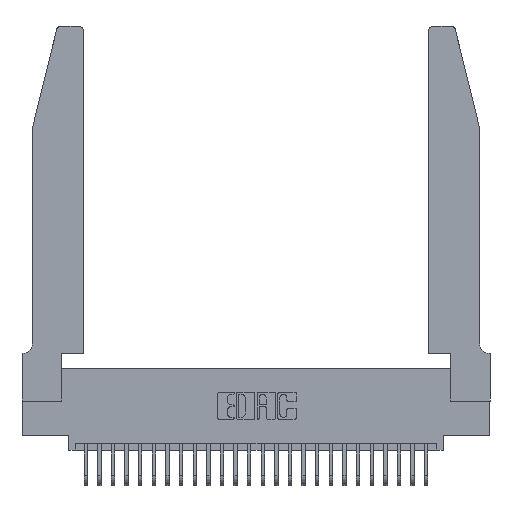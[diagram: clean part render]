
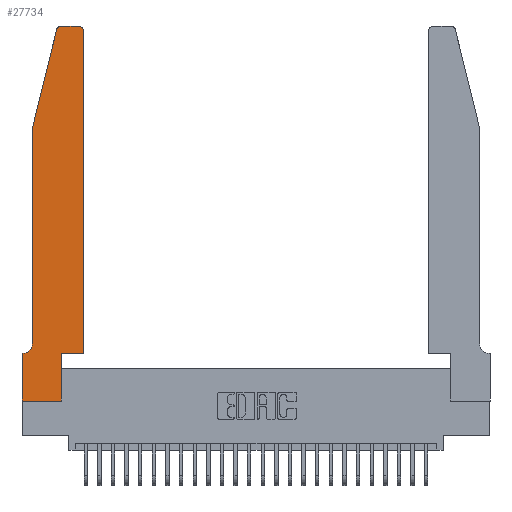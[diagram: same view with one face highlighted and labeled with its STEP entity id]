
A CAD part, top view. The second image highlights one B-rep face of the part: STEP entity #27734.
In plain terms, the highlighted planar face has unit normal (0, 0, 1).
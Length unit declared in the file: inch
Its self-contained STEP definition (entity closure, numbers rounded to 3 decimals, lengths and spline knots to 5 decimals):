
#188 = EDGE_CURVE ( 'NONE', #1949, #13038, #5815, .T. ) ;
#368 = LINE ( 'NONE', #1535, #14777 ) ;
#402 = CARTESIAN_POINT ( 'NONE',  ( 0.284, 2.75, 0.37 ) ) ;
#468 = AXIS2_PLACEMENT_3D ( 'NONE', #26087, #23922, #5599 ) ;
#580 = VERTEX_POINT ( 'NONE', #15066 ) ;
#971 = EDGE_LOOP ( 'NONE', ( #29012, #3470, #9494, #10318, #1989, #13173, #22170, #10500, #11775, #2356, #22865, #12247 ) ) ;
#1535 = CARTESIAN_POINT ( 'NONE',  ( 0., 0., 0.37 ) ) ;
#1949 = VERTEX_POINT ( 'NONE', #21469 ) ;
#1989 = ORIENTED_EDGE ( 'NONE', *, *, #4309, .T. ) ;
#2356 = ORIENTED_EDGE ( 'NONE', *, *, #188, .T. ) ;
#2629 = VERTEX_POINT ( 'NONE', #17180 ) ;
#3470 = ORIENTED_EDGE ( 'NONE', *, *, #5181, .T. ) ;
#3685 = LINE ( 'NONE', #28762, #26917 ) ;
#4158 = CARTESIAN_POINT ( 'NONE',  ( 0.0755, 2., 0.37 ) ) ;
#4309 = EDGE_CURVE ( 'NONE', #28322, #2629, #20389, .T. ) ;
#4954 = LINE ( 'NONE', #6471, #23658 ) ;
#5181 = EDGE_CURVE ( 'NONE', #15229, #28663, #14714, .T. ) ;
#5599 = DIRECTION ( 'NONE',  ( 1., 0., 0. ) ) ;
#5815 = LINE ( 'NONE', #12163, #25222 ) ;
#5998 = LINE ( 'NONE', #17079, #19383 ) ;
#6321 = DIRECTION ( 'NONE',  ( 0., 1., 0. ) ) ;
#6471 = CARTESIAN_POINT ( 'NONE',  ( 0.2605, 2.75, 0.37 ) ) ;
#6510 = CARTESIAN_POINT ( 'NONE',  ( 0.4205, 2.75, 0.37 ) ) ;
#6625 = EDGE_CURVE ( 'NONE', #580, #1949, #25628, .T. ) ;
#6723 = VECTOR ( 'NONE', #28165, 39.37008 ) ;
#7209 = CARTESIAN_POINT ( 'NONE',  ( 0.4205, 2.72, 0.37 ) ) ;
#8402 = EDGE_CURVE ( 'NONE', #13038, #26579, #3685, .T. ) ;
#8493 = FACE_OUTER_BOUND ( 'NONE', #971, .T. ) ;
#9494 = ORIENTED_EDGE ( 'NONE', *, *, #10702, .T. ) ;
#9653 = LINE ( 'NONE', #10586, #14929 ) ;
#10318 = ORIENTED_EDGE ( 'NONE', *, *, #11424, .T. ) ;
#10500 = ORIENTED_EDGE ( 'NONE', *, *, #14717, .T. ) ;
#10586 = CARTESIAN_POINT ( 'NONE',  ( 0., 0., 0.37 ) ) ;
#10702 = EDGE_CURVE ( 'NONE', #28663, #10866, #26811, .T. ) ;
#10866 = VERTEX_POINT ( 'NONE', #4158 ) ;
#11424 = EDGE_CURVE ( 'NONE', #10866, #28322, #5998, .T. ) ;
#11775 = ORIENTED_EDGE ( 'NONE', *, *, #6625, .T. ) ;
#11971 = DIRECTION ( 'NONE',  ( 0., 1., 0. ) ) ;
#12163 = CARTESIAN_POINT ( 'NONE',  ( 0.4505, 0.35, 0.37 ) ) ;
#12247 = ORIENTED_EDGE ( 'NONE', *, *, #17225, .T. ) ;
#12676 = CARTESIAN_POINT ( 'NONE',  ( 0.0755, 0.42, 0.37 ) ) ;
#13038 = VERTEX_POINT ( 'NONE', #16022 ) ;
#13173 = ORIENTED_EDGE ( 'NONE', *, *, #20077, .T. ) ;
#13421 = AXIS2_PLACEMENT_3D ( 'NONE', #7209, #18740, #27597 ) ;
#14231 = VERTEX_POINT ( 'NONE', #6510 ) ;
#14714 = CIRCLE ( 'NONE', #24878, 0.03 ) ;
#14717 = EDGE_CURVE ( 'NONE', #21330, #580, #368, .T. ) ;
#14777 = VECTOR ( 'NONE', #17518, 39.37008 ) ;
#14929 = VECTOR ( 'NONE', #19219, 39.37008 ) ;
#15066 = CARTESIAN_POINT ( 'NONE',  ( 0.2865, 0., 0.37 ) ) ;
#15229 = VERTEX_POINT ( 'NONE', #402 ) ;
#15526 = DIRECTION ( 'NONE',  ( -1., 0., 0. ) ) ;
#15791 = DIRECTION ( 'NONE',  ( 0., 0., 1. ) ) ;
#16022 = CARTESIAN_POINT ( 'NONE',  ( 0.4505, 0.35, 0.37 ) ) ;
#16034 = VERTEX_POINT ( 'NONE', #25802 ) ;
#16269 = DIRECTION ( 'NONE',  ( 1., 0., 0. ) ) ;
#17079 = CARTESIAN_POINT ( 'NONE',  ( 0.0755, 2., 0.37 ) ) ;
#17180 = CARTESIAN_POINT ( 'NONE',  ( 0.0055, 0.35, 0.37 ) ) ;
#17225 = EDGE_CURVE ( 'NONE', #26579, #14231, #18192, .T. ) ;
#17518 = DIRECTION ( 'NONE',  ( 1., 0., 0. ) ) ;
#18192 = CIRCLE ( 'NONE', #13421, 0.03 ) ;
#18740 = DIRECTION ( 'NONE',  ( 0., 0., 1. ) ) ;
#19219 = DIRECTION ( 'NONE',  ( 0., -1., 0. ) ) ;
#19383 = VECTOR ( 'NONE', #21771, 39.37008 ) ;
#19688 = LINE ( 'NONE', #27472, #22152 ) ;
#20077 = EDGE_CURVE ( 'NONE', #2629, #16034, #19688, .T. ) ;
#20389 = CIRCLE ( 'NONE', #21838, 0.07 ) ;
#20539 = CARTESIAN_POINT ( 'NONE',  ( 0.0755, 2., 0.37 ) ) ;
#20671 = VECTOR ( 'NONE', #11971, 39.37008 ) ;
#21330 = VERTEX_POINT ( 'NONE', #27000 ) ;
#21469 = CARTESIAN_POINT ( 'NONE',  ( 0.2865, 0.35, 0.37 ) ) ;
#21521 = DIRECTION ( 'NONE',  ( -1., 0., 0. ) ) ;
#21628 = CARTESIAN_POINT ( 'NONE',  ( 0.0055, 0.42, 0.37 ) ) ;
#21771 = DIRECTION ( 'NONE',  ( 0., -1., 0. ) ) ;
#21838 = AXIS2_PLACEMENT_3D ( 'NONE', #21628, #24008, #21521 ) ;
#22152 = VECTOR ( 'NONE', #25044, 39.37008 ) ;
#22170 = ORIENTED_EDGE ( 'NONE', *, *, #26011, .T. ) ;
#22609 = DIRECTION ( 'NONE',  ( 1., 0., 0. ) ) ;
#22865 = ORIENTED_EDGE ( 'NONE', *, *, #8402, .T. ) ;
#23483 = CARTESIAN_POINT ( 'NONE',  ( 0.2865, 0.35, 0.37 ) ) ;
#23658 = VECTOR ( 'NONE', #15526, 39.37008 ) ;
#23824 = PLANE ( 'NONE',  #468 ) ;
#23922 = DIRECTION ( 'NONE',  ( 0., 0., 1. ) ) ;
#24008 = DIRECTION ( 'NONE',  ( 0., 0., -1. ) ) ;
#24878 = AXIS2_PLACEMENT_3D ( 'NONE', #29094, #15791, #22609 ) ;
#25044 = DIRECTION ( 'NONE',  ( -1., 0., 0. ) ) ;
#25222 = VECTOR ( 'NONE', #16269, 39.37008 ) ;
#25628 = LINE ( 'NONE', #23483, #20671 ) ;
#25802 = CARTESIAN_POINT ( 'NONE',  ( 0., 0.35, 0.37 ) ) ;
#26011 = EDGE_CURVE ( 'NONE', #16034, #21330, #9653, .T. ) ;
#26087 = CARTESIAN_POINT ( 'NONE',  ( 0., 0.35, 0.37 ) ) ;
#26579 = VERTEX_POINT ( 'NONE', #27937 ) ;
#26811 = LINE ( 'NONE', #20539, #6723 ) ;
#26917 = VECTOR ( 'NONE', #6321, 39.37008 ) ;
#27000 = CARTESIAN_POINT ( 'NONE',  ( 0., 0., 0.37 ) ) ;
#27009 = CARTESIAN_POINT ( 'NONE',  ( 0.25487, 2.72718, 0.37 ) ) ;
#27472 = CARTESIAN_POINT ( 'NONE',  ( 0.0755, 0.35, 0.37 ) ) ;
#27597 = DIRECTION ( 'NONE',  ( 1., 0., 0. ) ) ;
#27734 = ADVANCED_FACE ( 'NONE', ( #8493 ), #23824, .T. ) ;
#27933 = EDGE_CURVE ( 'NONE', #14231, #15229, #4954, .T. ) ;
#27937 = CARTESIAN_POINT ( 'NONE',  ( 0.4505, 2.72, 0.37 ) ) ;
#28165 = DIRECTION ( 'NONE',  ( -0.239, -0.971, 0. ) ) ;
#28322 = VERTEX_POINT ( 'NONE', #12676 ) ;
#28663 = VERTEX_POINT ( 'NONE', #27009 ) ;
#28762 = CARTESIAN_POINT ( 'NONE',  ( 0.4505, 0.35, 0.37 ) ) ;
#29012 = ORIENTED_EDGE ( 'NONE', *, *, #27933, .T. ) ;
#29094 = CARTESIAN_POINT ( 'NONE',  ( 0.284, 2.72, 0.37 ) ) ;
